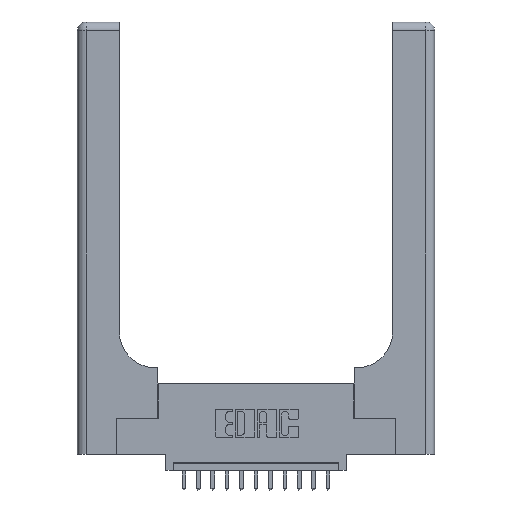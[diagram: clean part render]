
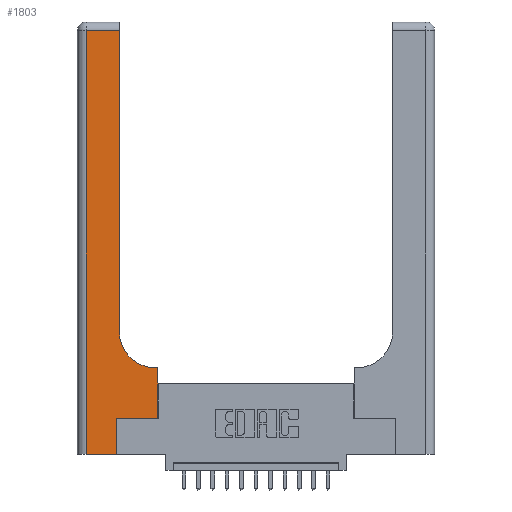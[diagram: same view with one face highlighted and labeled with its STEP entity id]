
A CAD part, top view. The second image highlights one B-rep face of the part: STEP entity #1803.
In plain terms, the highlighted planar face has unit normal (0, 0, 1).
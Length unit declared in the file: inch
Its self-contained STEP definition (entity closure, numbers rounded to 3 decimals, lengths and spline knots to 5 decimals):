
#141 = VECTOR ( 'NONE', #9595, 39.37008 ) ;
#409 = CARTESIAN_POINT ( 'NONE',  ( 0.06, 2.94, 0.37 ) ) ;
#684 = LINE ( 'NONE', #11942, #14710 ) ;
#985 = LINE ( 'NONE', #15057, #141 ) ;
#1080 = CARTESIAN_POINT ( 'NONE',  ( 0., 0., 0.37 ) ) ;
#1281 = DIRECTION ( 'NONE',  ( -1., 0., 0. ) ) ;
#1402 = ORIENTED_EDGE ( 'NONE', *, *, #2125, .T. ) ;
#1574 = VERTEX_POINT ( 'NONE', #3739 ) ;
#1803 = ADVANCED_FACE ( 'NONE', ( #9830 ), #2629, .F. ) ;
#1815 = DIRECTION ( 'NONE',  ( -1., 0., 0. ) ) ;
#2027 = VECTOR ( 'NONE', #1815, 39.37008 ) ;
#2125 = EDGE_CURVE ( 'NONE', #13977, #11657, #8697, .T. ) ;
#2204 = DIRECTION ( 'NONE',  ( -1., 0., 0. ) ) ;
#2629 = PLANE ( 'NONE',  #13104 ) ;
#2829 = ORIENTED_EDGE ( 'NONE', *, *, #10282, .T. ) ;
#3148 = VECTOR ( 'NONE', #13957, 39.37008 ) ;
#3244 = ORIENTED_EDGE ( 'NONE', *, *, #11028, .T. ) ;
#3262 = VECTOR ( 'NONE', #12247, 39.37008 ) ;
#3406 = CARTESIAN_POINT ( 'NONE',  ( 0.269, 0.25, 0.37 ) ) ;
#3452 = ORIENTED_EDGE ( 'NONE', *, *, #9000, .T. ) ;
#3666 = CARTESIAN_POINT ( 'NONE',  ( 0.06, 0., 0.37 ) ) ;
#3716 = CIRCLE ( 'NONE', #15282, 0.25 ) ;
#3739 = CARTESIAN_POINT ( 'NONE',  ( 0.2915, 2.94, 0.37 ) ) ;
#3768 = VERTEX_POINT ( 'NONE', #8190 ) ;
#4190 = EDGE_CURVE ( 'NONE', #1574, #10878, #17626, .T. ) ;
#5320 = CARTESIAN_POINT ( 'NONE',  ( 0.2915, 3., 0.37 ) ) ;
#5377 = DIRECTION ( 'NONE',  ( 0., 0., -1. ) ) ;
#5549 = ORIENTED_EDGE ( 'NONE', *, *, #10420, .T. ) ;
#5651 = LINE ( 'NONE', #10882, #3262 ) ;
#5900 = DIRECTION ( 'NONE',  ( 0., 0., -1. ) ) ;
#6249 = CARTESIAN_POINT ( 'NONE',  ( 0., 2.94, 0.37 ) ) ;
#6307 = CARTESIAN_POINT ( 'NONE',  ( 0.2915, 0.85, 0.37 ) ) ;
#6854 = EDGE_CURVE ( 'NONE', #9924, #9388, #985, .T. ) ;
#6862 = LINE ( 'NONE', #13784, #3148 ) ;
#6966 = VERTEX_POINT ( 'NONE', #8662 ) ;
#7082 = ORIENTED_EDGE ( 'NONE', *, *, #4190, .T. ) ;
#7388 = CARTESIAN_POINT ( 'NONE',  ( 0.5585, 0.25, 0.37 ) ) ;
#8190 = CARTESIAN_POINT ( 'NONE',  ( 0.5415, 0.6, 0.37 ) ) ;
#8296 = VECTOR ( 'NONE', #9599, 39.37008 ) ;
#8662 = CARTESIAN_POINT ( 'NONE',  ( 0.5585, 0.6, 0.37 ) ) ;
#8697 = LINE ( 'NONE', #1080, #8296 ) ;
#8761 = DIRECTION ( 'NONE',  ( 1., 0., 0. ) ) ;
#8960 = EDGE_LOOP ( 'NONE', ( #3244, #7082, #11302, #1402, #13379, #14448, #5549, #3452, #2829 ) ) ;
#9000 = EDGE_CURVE ( 'NONE', #6966, #3768, #11096, .T. ) ;
#9388 = VERTEX_POINT ( 'NONE', #7388 ) ;
#9595 = DIRECTION ( 'NONE',  ( 1., 0., 0. ) ) ;
#9599 = DIRECTION ( 'NONE',  ( 1., 0., 0. ) ) ;
#9830 = FACE_OUTER_BOUND ( 'NONE', #8960, .T. ) ;
#9924 = VERTEX_POINT ( 'NONE', #3406 ) ;
#10282 = EDGE_CURVE ( 'NONE', #3768, #13330, #3716, .T. ) ;
#10340 = CARTESIAN_POINT ( 'NONE',  ( 0.2915, 0.6, 0.37 ) ) ;
#10420 = EDGE_CURVE ( 'NONE', #9388, #6966, #5651, .T. ) ;
#10878 = VERTEX_POINT ( 'NONE', #409 ) ;
#10882 = CARTESIAN_POINT ( 'NONE',  ( 0.5585, 0.25, 0.37 ) ) ;
#11028 = EDGE_CURVE ( 'NONE', #13330, #1574, #14016, .T. ) ;
#11096 = LINE ( 'NONE', #10340, #2027 ) ;
#11302 = ORIENTED_EDGE ( 'NONE', *, *, #15757, .T. ) ;
#11657 = VERTEX_POINT ( 'NONE', #13965 ) ;
#11942 = CARTESIAN_POINT ( 'NONE',  ( 0.06, 3., 0.37 ) ) ;
#11955 = DIRECTION ( 'NONE',  ( 0., 1., 0. ) ) ;
#12247 = DIRECTION ( 'NONE',  ( 0., 1., 0. ) ) ;
#12738 = CARTESIAN_POINT ( 'NONE',  ( 0.5415, 0.85, 0.37 ) ) ;
#13104 = AXIS2_PLACEMENT_3D ( 'NONE', #13617, #5377, #1281 ) ;
#13330 = VERTEX_POINT ( 'NONE', #6307 ) ;
#13379 = ORIENTED_EDGE ( 'NONE', *, *, #14434, .T. ) ;
#13617 = CARTESIAN_POINT ( 'NONE',  ( 0., 3., 0.37 ) ) ;
#13784 = CARTESIAN_POINT ( 'NONE',  ( 0.269, 0., 0.37 ) ) ;
#13957 = DIRECTION ( 'NONE',  ( 0., 1., 0. ) ) ;
#13965 = CARTESIAN_POINT ( 'NONE',  ( 0.269, 0., 0.37 ) ) ;
#13977 = VERTEX_POINT ( 'NONE', #3666 ) ;
#14016 = LINE ( 'NONE', #5320, #15960 ) ;
#14434 = EDGE_CURVE ( 'NONE', #11657, #9924, #6862, .T. ) ;
#14448 = ORIENTED_EDGE ( 'NONE', *, *, #6854, .T. ) ;
#14710 = VECTOR ( 'NONE', #17230, 39.37008 ) ;
#15057 = CARTESIAN_POINT ( 'NONE',  ( 0.269, 0.25, 0.37 ) ) ;
#15058 = VECTOR ( 'NONE', #2204, 39.37008 ) ;
#15282 = AXIS2_PLACEMENT_3D ( 'NONE', #12738, #5900, #8761 ) ;
#15757 = EDGE_CURVE ( 'NONE', #10878, #13977, #684, .T. ) ;
#15960 = VECTOR ( 'NONE', #11955, 39.37008 ) ;
#17230 = DIRECTION ( 'NONE',  ( 0., -1., 0. ) ) ;
#17626 = LINE ( 'NONE', #6249, #15058 ) ;
